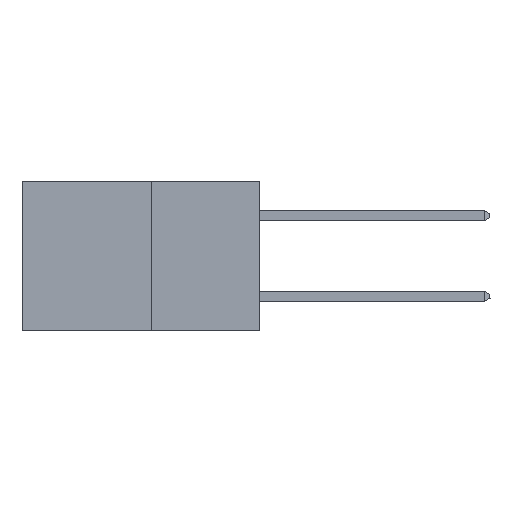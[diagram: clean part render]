
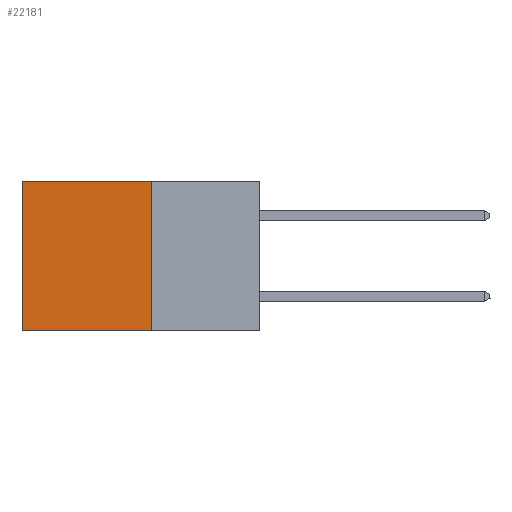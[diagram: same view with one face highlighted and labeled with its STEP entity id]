
A CAD part, left-side view. The second image highlights one B-rep face of the part: STEP entity #22181.
In plain terms, the highlighted planar face has unit normal (-1, 0, 0).
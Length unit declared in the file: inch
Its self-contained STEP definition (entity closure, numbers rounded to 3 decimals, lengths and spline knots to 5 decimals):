
#301 = ORIENTED_EDGE ( 'NONE', *, *, #19535, .T. ) ;
#990 = VECTOR ( 'NONE', #26606, 39.37008 ) ;
#2212 = VECTOR ( 'NONE', #14590, 39.37008 ) ;
#2500 = LINE ( 'NONE', #21655, #990 ) ;
#2535 = VERTEX_POINT ( 'NONE', #11687 ) ;
#4736 = CARTESIAN_POINT ( 'NONE',  ( 0.277, 0.59, 0. ) ) ;
#4752 = CARTESIAN_POINT ( 'NONE',  ( 0.277, 0.59, -0.37 ) ) ;
#5633 = ORIENTED_EDGE ( 'NONE', *, *, #28143, .T. ) ;
#7419 = CARTESIAN_POINT ( 'NONE',  ( 0.277, 0.27, -0.37 ) ) ;
#8238 = CARTESIAN_POINT ( 'NONE',  ( 0.277, 0.27, -0.37 ) ) ;
#8999 = VERTEX_POINT ( 'NONE', #4736 ) ;
#9522 = ORIENTED_EDGE ( 'NONE', *, *, #15595, .F. ) ;
#9855 = DIRECTION ( 'NONE',  ( 0., 1., 0. ) ) ;
#10684 = DIRECTION ( 'NONE',  ( 0., 0., -1. ) ) ;
#11687 = CARTESIAN_POINT ( 'NONE',  ( 0.277, 0.27, -0.37 ) ) ;
#12131 = CARTESIAN_POINT ( 'NONE',  ( 0.277, 0.59, -0.37 ) ) ;
#13837 = CARTESIAN_POINT ( 'NONE',  ( 0.277, 0.27, 0. ) ) ;
#14018 = VECTOR ( 'NONE', #27851, 39.37008 ) ;
#14590 = DIRECTION ( 'NONE',  ( 0., 0., -1. ) ) ;
#15217 = LINE ( 'NONE', #12131, #2212 ) ;
#15466 = CARTESIAN_POINT ( 'NONE',  ( 0.277, 0.27, -0.37 ) ) ;
#15503 = ORIENTED_EDGE ( 'NONE', *, *, #20753, .F. ) ;
#15595 = EDGE_CURVE ( 'NONE', #2535, #25248, #25593, .T. ) ;
#17392 = EDGE_LOOP ( 'NONE', ( #301, #9522, #15503, #5633 ) ) ;
#17952 = PLANE ( 'NONE',  #25490 ) ;
#18555 = FACE_OUTER_BOUND ( 'NONE', #17392, .T. ) ;
#19535 = EDGE_CURVE ( 'NONE', #8999, #25248, #15217, .T. ) ;
#20545 = LINE ( 'NONE', #15466, #14018 ) ;
#20753 = EDGE_CURVE ( 'NONE', #21688, #2535, #20545, .T. ) ;
#21655 = CARTESIAN_POINT ( 'NONE',  ( 0.277, 0.27, 0. ) ) ;
#21688 = VERTEX_POINT ( 'NONE', #13837 ) ;
#22181 = ADVANCED_FACE ( 'NONE', ( #18555 ), #17952, .F. ) ;
#24813 = VECTOR ( 'NONE', #9855, 39.37008 ) ;
#25248 = VERTEX_POINT ( 'NONE', #4752 ) ;
#25408 = DIRECTION ( 'NONE',  ( 1., 0., 0. ) ) ;
#25490 = AXIS2_PLACEMENT_3D ( 'NONE', #8238, #25408, #10684 ) ;
#25593 = LINE ( 'NONE', #7419, #24813 ) ;
#26606 = DIRECTION ( 'NONE',  ( 0., 1., 0. ) ) ;
#27851 = DIRECTION ( 'NONE',  ( 0., 0., -1. ) ) ;
#28143 = EDGE_CURVE ( 'NONE', #21688, #8999, #2500, .T. ) ;
